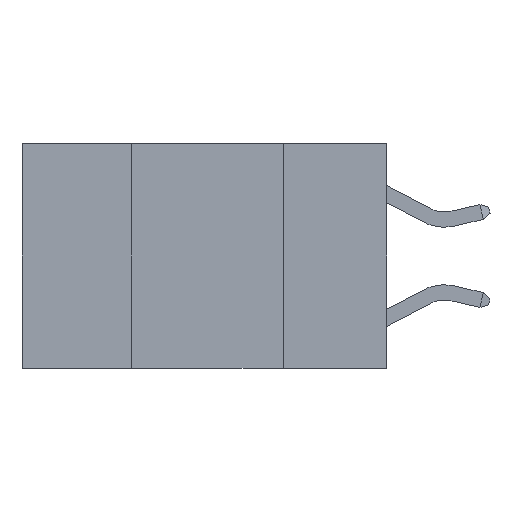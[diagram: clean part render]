
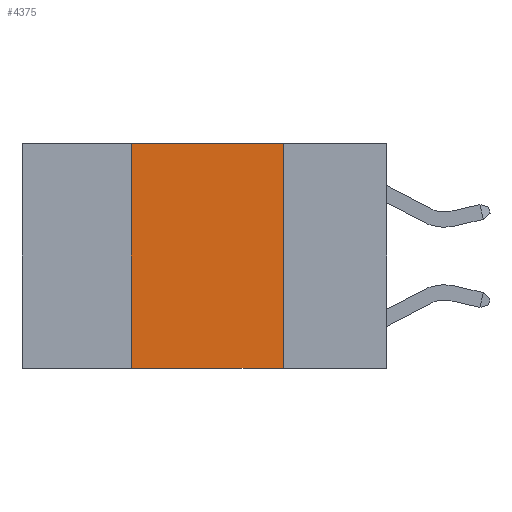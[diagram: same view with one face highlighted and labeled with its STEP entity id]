
A CAD part, left-side view. The second image highlights one B-rep face of the part: STEP entity #4375.
In plain terms, the highlighted planar face has unit normal (-1, 0, 0).
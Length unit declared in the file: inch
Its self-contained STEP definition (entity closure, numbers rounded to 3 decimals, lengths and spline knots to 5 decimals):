
#465 = ORIENTED_EDGE ( 'NONE', *, *, #9315, .T. ) ;
#531 = ORIENTED_EDGE ( 'NONE', *, *, #11014, .F. ) ;
#616 = CARTESIAN_POINT ( 'NONE',  ( 0., 0.42, 0. ) ) ;
#760 = CARTESIAN_POINT ( 'NONE',  ( 0., 0.17, 0. ) ) ;
#808 = EDGE_CURVE ( 'NONE', #3084, #1200, #3482, .T. ) ;
#812 = CARTESIAN_POINT ( 'NONE',  ( 0., 0.42, 0. ) ) ;
#1200 = VERTEX_POINT ( 'NONE', #812 ) ;
#1635 = DIRECTION ( 'NONE',  ( 0., -1., 0. ) ) ;
#1693 = LINE ( 'NONE', #10545, #9509 ) ;
#2768 = VERTEX_POINT ( 'NONE', #4540 ) ;
#2914 = VECTOR ( 'NONE', #7012, 39.37008 ) ;
#3050 = CARTESIAN_POINT ( 'NONE',  ( 0., 0.6, 0. ) ) ;
#3069 = CARTESIAN_POINT ( 'NONE',  ( 0., 0.6, -0.37 ) ) ;
#3084 = VERTEX_POINT ( 'NONE', #8463 ) ;
#3482 = LINE ( 'NONE', #616, #2914 ) ;
#3847 = PLANE ( 'NONE',  #6642 ) ;
#4375 = ADVANCED_FACE ( 'NONE', ( #4964 ), #3847, .F. ) ;
#4540 = CARTESIAN_POINT ( 'NONE',  ( 0., 0.17, -0.37 ) ) ;
#4964 = FACE_OUTER_BOUND ( 'NONE', #5154, .T. ) ;
#5154 = EDGE_LOOP ( 'NONE', ( #11097, #531, #9214, #465 ) ) ;
#5794 = LINE ( 'NONE', #3069, #9477 ) ;
#6118 = VECTOR ( 'NONE', #10365, 39.37008 ) ;
#6238 = EDGE_CURVE ( 'NONE', #6612, #2768, #7731, .T. ) ;
#6612 = VERTEX_POINT ( 'NONE', #9033 ) ;
#6642 = AXIS2_PLACEMENT_3D ( 'NONE', #3050, #9968, #10020 ) ;
#7012 = DIRECTION ( 'NONE',  ( 0., 0., 1. ) ) ;
#7731 = LINE ( 'NONE', #760, #6118 ) ;
#8463 = CARTESIAN_POINT ( 'NONE',  ( 0., 0.42, -0.37 ) ) ;
#9033 = CARTESIAN_POINT ( 'NONE',  ( 0., 0.17, 0. ) ) ;
#9214 = ORIENTED_EDGE ( 'NONE', *, *, #808, .F. ) ;
#9315 = EDGE_CURVE ( 'NONE', #3084, #2768, #5794, .T. ) ;
#9382 = DIRECTION ( 'NONE',  ( 0., -1., 0. ) ) ;
#9477 = VECTOR ( 'NONE', #9382, 39.37008 ) ;
#9509 = VECTOR ( 'NONE', #1635, 39.37008 ) ;
#9968 = DIRECTION ( 'NONE',  ( 1., 0., 0. ) ) ;
#10020 = DIRECTION ( 'NONE',  ( 0., 0., -1. ) ) ;
#10365 = DIRECTION ( 'NONE',  ( 0., 0., -1. ) ) ;
#10545 = CARTESIAN_POINT ( 'NONE',  ( 0., 0.6, 0. ) ) ;
#11014 = EDGE_CURVE ( 'NONE', #1200, #6612, #1693, .T. ) ;
#11097 = ORIENTED_EDGE ( 'NONE', *, *, #6238, .F. ) ;
